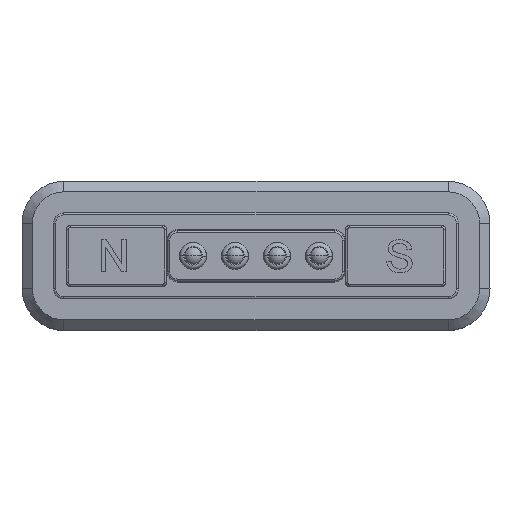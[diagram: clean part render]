
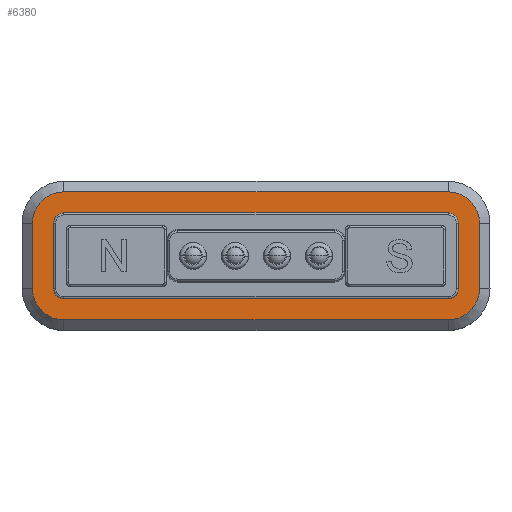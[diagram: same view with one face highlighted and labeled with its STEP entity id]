
A CAD part, top view. The second image highlights one B-rep face of the part: STEP entity #6380.
In plain terms, the highlighted planar face has unit normal (0, 0, 1).
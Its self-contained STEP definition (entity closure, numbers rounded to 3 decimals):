
#117 = CIRCLE ( 'NONE', #8802, 0.5 ) ;
#155 = DIRECTION ( 'NONE',  ( -1., 0., 0. ) ) ;
#257 = VERTEX_POINT ( 'NONE', #4176 ) ;
#275 = CIRCLE ( 'NONE', #6792, 0.5 ) ;
#291 = EDGE_CURVE ( 'NONE', #10011, #7267, #2291, .T. ) ;
#338 = AXIS2_PLACEMENT_3D ( 'NONE', #2332, #540, #1584 ) ;
#361 = CARTESIAN_POINT ( 'NONE',  ( 9.15, 1.55, -0.5 ) ) ;
#382 = CARTESIAN_POINT ( 'NONE',  ( 10.65, 1.55, -0.5 ) ) ;
#540 = DIRECTION ( 'NONE',  ( 0., 0., 1. ) ) ;
#559 = EDGE_CURVE ( 'NONE', #5677, #4583, #2933, .T. ) ;
#578 = ORIENTED_EDGE ( 'NONE', *, *, #11304, .T. ) ;
#721 = CARTESIAN_POINT ( 'NONE',  ( -9.15, 1.55, -0.5 ) ) ;
#724 = ORIENTED_EDGE ( 'NONE', *, *, #10160, .T. ) ;
#925 = EDGE_CURVE ( 'NONE', #10699, #6998, #5624, .T. ) ;
#977 = LINE ( 'NONE', #1967, #10610 ) ;
#1132 = ORIENTED_EDGE ( 'NONE', *, *, #5200, .F. ) ;
#1210 = CARTESIAN_POINT ( 'NONE',  ( 9.15, 3.05, -0.5 ) ) ;
#1268 = DIRECTION ( 'NONE',  ( 0., 1., 0. ) ) ;
#1289 = DIRECTION ( 'NONE',  ( 0., 0., 1. ) ) ;
#1353 = DIRECTION ( 'NONE',  ( 1., 0., 0. ) ) ;
#1409 = CARTESIAN_POINT ( 'NONE',  ( -9.15, 3.05, -0.5 ) ) ;
#1422 = CARTESIAN_POINT ( 'NONE',  ( -9.15, -3.05, -0.5 ) ) ;
#1584 = DIRECTION ( 'NONE',  ( 0., 1., 0. ) ) ;
#1623 = VERTEX_POINT ( 'NONE', #11129 ) ;
#1631 = DIRECTION ( 'NONE',  ( 0., -1., 0. ) ) ;
#1640 = CIRCLE ( 'NONE', #10934, 0.5 ) ;
#1752 = ORIENTED_EDGE ( 'NONE', *, *, #559, .F. ) ;
#1867 = CARTESIAN_POINT ( 'NONE',  ( -9.15, -1.55, -0.5 ) ) ;
#1906 = DIRECTION ( 'NONE',  ( 0., -1., 0. ) ) ;
#1955 = CARTESIAN_POINT ( 'NONE',  ( 9.15, 2.05, -0.5 ) ) ;
#1967 = CARTESIAN_POINT ( 'NONE',  ( 9.65, -1.55, -0.5 ) ) ;
#2019 = DIRECTION ( 'NONE',  ( -1., 0., 0. ) ) ;
#2151 = AXIS2_PLACEMENT_3D ( 'NONE', #721, #8460, #2019 ) ;
#2226 = CARTESIAN_POINT ( 'NONE',  ( 9.15, -1.55, -0.5 ) ) ;
#2291 = LINE ( 'NONE', #4231, #4692 ) ;
#2332 = CARTESIAN_POINT ( 'NONE',  ( -9.15, 1.55, -0.5 ) ) ;
#2356 = VERTEX_POINT ( 'NONE', #1210 ) ;
#2364 = DIRECTION ( 'NONE',  ( 0., 0., -1. ) ) ;
#2449 = EDGE_CURVE ( 'NONE', #4993, #10867, #8638, .T. ) ;
#2456 = EDGE_CURVE ( 'NONE', #5677, #12223, #275, .T. ) ;
#2640 = VERTEX_POINT ( 'NONE', #10984 ) ;
#2664 = EDGE_CURVE ( 'NONE', #4993, #6998, #5221, .T. ) ;
#2860 = DIRECTION ( 'NONE',  ( -1., 0., 0. ) ) ;
#2933 = LINE ( 'NONE', #4684, #8601 ) ;
#3014 = DIRECTION ( 'NONE',  ( -1., 0., 0. ) ) ;
#3081 = CARTESIAN_POINT ( 'NONE',  ( -10.65, -1.55, -0.5 ) ) ;
#3160 = ORIENTED_EDGE ( 'NONE', *, *, #7298, .F. ) ;
#3335 = DIRECTION ( 'NONE',  ( 1., 0., 0. ) ) ;
#3546 = CARTESIAN_POINT ( 'NONE',  ( 9.65, 1.55, -0.5 ) ) ;
#3664 = AXIS2_PLACEMENT_3D ( 'NONE', #10825, #1289, #1353 ) ;
#3892 = LINE ( 'NONE', #8649, #8135 ) ;
#3957 = EDGE_CURVE ( 'NONE', #4235, #1623, #117, .T. ) ;
#4007 = EDGE_LOOP ( 'NONE', ( #4962, #9969, #8797, #1752, #5936, #1132, #10568, #3160 ) ) ;
#4063 = DIRECTION ( 'NONE',  ( 0., -1., 0. ) ) ;
#4176 = CARTESIAN_POINT ( 'NONE',  ( -9.15, 3.05, -0.5 ) ) ;
#4231 = CARTESIAN_POINT ( 'NONE',  ( -10.65, 1.55, -0.5 ) ) ;
#4235 = VERTEX_POINT ( 'NONE', #5961 ) ;
#4267 = AXIS2_PLACEMENT_3D ( 'NONE', #361, #9939, #6104 ) ;
#4326 = VECTOR ( 'NONE', #3014, 1000. ) ;
#4583 = VERTEX_POINT ( 'NONE', #12130 ) ;
#4633 = EDGE_LOOP ( 'NONE', ( #7651, #724, #10113, #8571, #7092, #10656, #9834, #578 ) ) ;
#4684 = CARTESIAN_POINT ( 'NONE',  ( 9.15, 2.05, -0.5 ) ) ;
#4692 = VECTOR ( 'NONE', #11784, 1000. ) ;
#4962 = ORIENTED_EDGE ( 'NONE', *, *, #3957, .T. ) ;
#4993 = VERTEX_POINT ( 'NONE', #7694 ) ;
#5065 = CARTESIAN_POINT ( 'NONE',  ( 9.15, 1.55, -0.5 ) ) ;
#5200 = EDGE_CURVE ( 'NONE', #11374, #12223, #977, .T. ) ;
#5221 = CIRCLE ( 'NONE', #7376, 1.5 ) ;
#5333 = CIRCLE ( 'NONE', #2151, 0.5 ) ;
#5545 = EDGE_CURVE ( 'NONE', #8597, #4583, #5333, .T. ) ;
#5624 = LINE ( 'NONE', #5692, #7940 ) ;
#5654 = DIRECTION ( 'NONE',  ( 0., 0., 1. ) ) ;
#5677 = VERTEX_POINT ( 'NONE', #1955 ) ;
#5692 = CARTESIAN_POINT ( 'NONE',  ( 10.65, 1.55, -0.5 ) ) ;
#5695 = LINE ( 'NONE', #9713, #11635 ) ;
#5816 = DIRECTION ( 'NONE',  ( 0., 1., 0. ) ) ;
#5936 = ORIENTED_EDGE ( 'NONE', *, *, #2456, .T. ) ;
#5961 = CARTESIAN_POINT ( 'NONE',  ( -9.15, -2.05, -0.5 ) ) ;
#5964 = EDGE_CURVE ( 'NONE', #11374, #2640, #1640, .T. ) ;
#6104 = DIRECTION ( 'NONE',  ( 1., 0., 0. ) ) ;
#6176 = CARTESIAN_POINT ( 'NONE',  ( -9.65, 1.55, -0.5 ) ) ;
#6240 = AXIS2_PLACEMENT_3D ( 'NONE', #1867, #5654, #2860 ) ;
#6292 = CARTESIAN_POINT ( 'NONE',  ( 9.65, -1.55, -0.5 ) ) ;
#6338 = CARTESIAN_POINT ( 'NONE',  ( 9.15, -1.55, -0.5 ) ) ;
#6380 = ADVANCED_FACE ( 'NONE', ( #7980, #9835 ), #9773, .T. ) ;
#6675 = DIRECTION ( 'NONE',  ( 0., -1., 0. ) ) ;
#6720 = EDGE_CURVE ( 'NONE', #10699, #2356, #11786, .T. ) ;
#6754 = DIRECTION ( 'NONE',  ( 0., 0., -1. ) ) ;
#6792 = AXIS2_PLACEMENT_3D ( 'NONE', #5065, #6970, #1268 ) ;
#6970 = DIRECTION ( 'NONE',  ( 0., 0., -1. ) ) ;
#6998 = VERTEX_POINT ( 'NONE', #11683 ) ;
#7077 = CARTESIAN_POINT ( 'NONE',  ( -9.15, -1.55, -0.5 ) ) ;
#7092 = ORIENTED_EDGE ( 'NONE', *, *, #925, .F. ) ;
#7267 = VERTEX_POINT ( 'NONE', #3081 ) ;
#7298 = EDGE_CURVE ( 'NONE', #4235, #2640, #3892, .T. ) ;
#7376 = AXIS2_PLACEMENT_3D ( 'NONE', #6338, #10112, #1631 ) ;
#7651 = ORIENTED_EDGE ( 'NONE', *, *, #291, .T. ) ;
#7694 = CARTESIAN_POINT ( 'NONE',  ( 9.15, -3.05, -0.5 ) ) ;
#7852 = DIRECTION ( 'NONE',  ( 1., 0., 0. ) ) ;
#7940 = VECTOR ( 'NONE', #6675, 1000. ) ;
#7980 = FACE_OUTER_BOUND ( 'NONE', #4633, .T. ) ;
#8135 = VECTOR ( 'NONE', #7852, 1000. ) ;
#8415 = EDGE_CURVE ( 'NONE', #8597, #1623, #5695, .T. ) ;
#8460 = DIRECTION ( 'NONE',  ( 0., 0., -1. ) ) ;
#8571 = ORIENTED_EDGE ( 'NONE', *, *, #2664, .T. ) ;
#8597 = VERTEX_POINT ( 'NONE', #6176 ) ;
#8601 = VECTOR ( 'NONE', #155, 1000. ) ;
#8638 = LINE ( 'NONE', #11505, #4326 ) ;
#8649 = CARTESIAN_POINT ( 'NONE',  ( -9.15, -2.05, -0.5 ) ) ;
#8743 = EDGE_CURVE ( 'NONE', #257, #2356, #10822, .T. ) ;
#8797 = ORIENTED_EDGE ( 'NONE', *, *, #5545, .T. ) ;
#8802 = AXIS2_PLACEMENT_3D ( 'NONE', #7077, #2364, #4063 ) ;
#9228 = VECTOR ( 'NONE', #3335, 1000. ) ;
#9713 = CARTESIAN_POINT ( 'NONE',  ( -9.65, 1.55, -0.5 ) ) ;
#9773 = PLANE ( 'NONE',  #3664 ) ;
#9834 = ORIENTED_EDGE ( 'NONE', *, *, #8743, .F. ) ;
#9835 = FACE_BOUND ( 'NONE', #4007, .T. ) ;
#9939 = DIRECTION ( 'NONE',  ( 0., 0., 1. ) ) ;
#9969 = ORIENTED_EDGE ( 'NONE', *, *, #8415, .F. ) ;
#10011 = VERTEX_POINT ( 'NONE', #10921 ) ;
#10112 = DIRECTION ( 'NONE',  ( 0., 0., 1. ) ) ;
#10113 = ORIENTED_EDGE ( 'NONE', *, *, #2449, .F. ) ;
#10160 = EDGE_CURVE ( 'NONE', #7267, #10867, #10796, .T. ) ;
#10469 = DIRECTION ( 'NONE',  ( 1., 0., 0. ) ) ;
#10568 = ORIENTED_EDGE ( 'NONE', *, *, #5964, .T. ) ;
#10610 = VECTOR ( 'NONE', #5816, 1000. ) ;
#10656 = ORIENTED_EDGE ( 'NONE', *, *, #6720, .T. ) ;
#10699 = VERTEX_POINT ( 'NONE', #382 ) ;
#10796 = CIRCLE ( 'NONE', #6240, 1.5 ) ;
#10822 = LINE ( 'NONE', #1409, #9228 ) ;
#10825 = CARTESIAN_POINT ( 'NONE',  ( 0., 0., -0.5 ) ) ;
#10867 = VERTEX_POINT ( 'NONE', #1422 ) ;
#10921 = CARTESIAN_POINT ( 'NONE',  ( -10.65, 1.55, -0.5 ) ) ;
#10934 = AXIS2_PLACEMENT_3D ( 'NONE', #2226, #6754, #10469 ) ;
#10984 = CARTESIAN_POINT ( 'NONE',  ( 9.15, -2.05, -0.5 ) ) ;
#11010 = CIRCLE ( 'NONE', #338, 1.5 ) ;
#11129 = CARTESIAN_POINT ( 'NONE',  ( -9.65, -1.55, -0.5 ) ) ;
#11304 = EDGE_CURVE ( 'NONE', #257, #10011, #11010, .T. ) ;
#11374 = VERTEX_POINT ( 'NONE', #6292 ) ;
#11505 = CARTESIAN_POINT ( 'NONE',  ( 9.15, -3.05, -0.5 ) ) ;
#11635 = VECTOR ( 'NONE', #1906, 1000. ) ;
#11683 = CARTESIAN_POINT ( 'NONE',  ( 10.65, -1.55, -0.5 ) ) ;
#11784 = DIRECTION ( 'NONE',  ( 0., -1., 0. ) ) ;
#11786 = CIRCLE ( 'NONE', #4267, 1.5 ) ;
#12130 = CARTESIAN_POINT ( 'NONE',  ( -9.15, 2.05, -0.5 ) ) ;
#12223 = VERTEX_POINT ( 'NONE', #3546 ) ;
